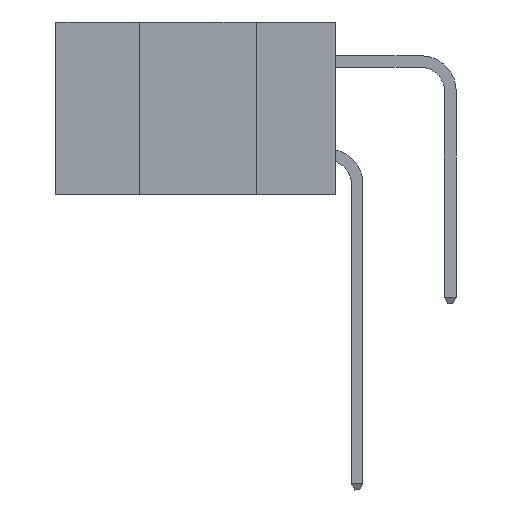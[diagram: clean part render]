
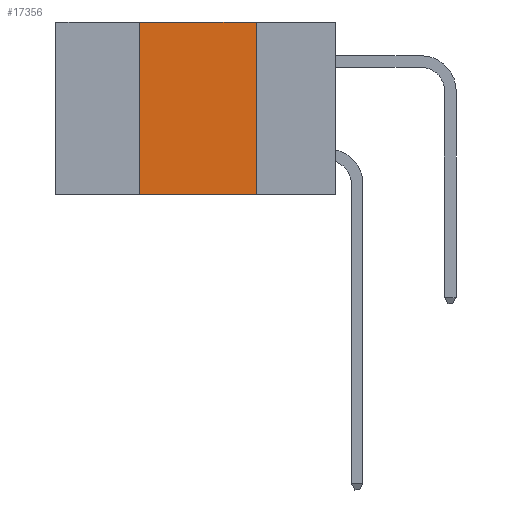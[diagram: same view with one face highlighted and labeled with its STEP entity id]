
A CAD part, left-side view. The second image highlights one B-rep face of the part: STEP entity #17356.
In plain terms, the highlighted planar face has unit normal (-1, 0, 0).
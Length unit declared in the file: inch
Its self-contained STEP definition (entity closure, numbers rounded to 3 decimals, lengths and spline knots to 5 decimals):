
#364 = ORIENTED_EDGE ( 'NONE', *, *, #7709, .F. ) ;
#2696 = VERTEX_POINT ( 'NONE', #29429 ) ;
#3356 = AXIS2_PLACEMENT_3D ( 'NONE', #24708, #15119, #13085 ) ;
#4903 = DIRECTION ( 'NONE',  ( 0., -1., 0. ) ) ;
#5418 = EDGE_CURVE ( 'NONE', #24026, #24353, #25997, .T. ) ;
#5653 = LINE ( 'NONE', #22115, #6762 ) ;
#6004 = VECTOR ( 'NONE', #18361, 39.37008 ) ;
#6762 = VECTOR ( 'NONE', #15137, 39.37008 ) ;
#7709 = EDGE_CURVE ( 'NONE', #16494, #24026, #5653, .T. ) ;
#8217 = EDGE_LOOP ( 'NONE', ( #12691, #22818, #364, #18234 ) ) ;
#8428 = EDGE_CURVE ( 'NONE', #24353, #2696, #9039, .T. ) ;
#9039 = LINE ( 'NONE', #13537, #9693 ) ;
#9693 = VECTOR ( 'NONE', #18511, 39.37008 ) ;
#10444 = FACE_OUTER_BOUND ( 'NONE', #8217, .T. ) ;
#11846 = VECTOR ( 'NONE', #4903, 39.37008 ) ;
#12134 = EDGE_CURVE ( 'NONE', #16494, #2696, #13717, .T. ) ;
#12691 = ORIENTED_EDGE ( 'NONE', *, *, #8428, .F. ) ;
#13085 = DIRECTION ( 'NONE',  ( 0., 0., -1. ) ) ;
#13537 = CARTESIAN_POINT ( 'NONE',  ( 0., 0.17, 0. ) ) ;
#13717 = LINE ( 'NONE', #18198, #6004 ) ;
#13809 = CARTESIAN_POINT ( 'NONE',  ( 0., 0.42, 0. ) ) ;
#15119 = DIRECTION ( 'NONE',  ( 1., 0., 0. ) ) ;
#15137 = DIRECTION ( 'NONE',  ( 0., 0., 1. ) ) ;
#15632 = CARTESIAN_POINT ( 'NONE',  ( 0., 0.17, 0. ) ) ;
#16494 = VERTEX_POINT ( 'NONE', #19579 ) ;
#17356 = ADVANCED_FACE ( 'NONE', ( #10444 ), #17446, .F. ) ;
#17446 = PLANE ( 'NONE',  #3356 ) ;
#18198 = CARTESIAN_POINT ( 'NONE',  ( 0., 0.6, -0.37 ) ) ;
#18234 = ORIENTED_EDGE ( 'NONE', *, *, #12134, .T. ) ;
#18361 = DIRECTION ( 'NONE',  ( 0., -1., 0. ) ) ;
#18511 = DIRECTION ( 'NONE',  ( 0., 0., -1. ) ) ;
#19034 = CARTESIAN_POINT ( 'NONE',  ( 0., 0.6, 0. ) ) ;
#19579 = CARTESIAN_POINT ( 'NONE',  ( 0., 0.42, -0.37 ) ) ;
#22115 = CARTESIAN_POINT ( 'NONE',  ( 0., 0.42, 0. ) ) ;
#22818 = ORIENTED_EDGE ( 'NONE', *, *, #5418, .F. ) ;
#24026 = VERTEX_POINT ( 'NONE', #13809 ) ;
#24353 = VERTEX_POINT ( 'NONE', #15632 ) ;
#24708 = CARTESIAN_POINT ( 'NONE',  ( 0., 0.6, 0. ) ) ;
#25997 = LINE ( 'NONE', #19034, #11846 ) ;
#29429 = CARTESIAN_POINT ( 'NONE',  ( 0., 0.17, -0.37 ) ) ;
